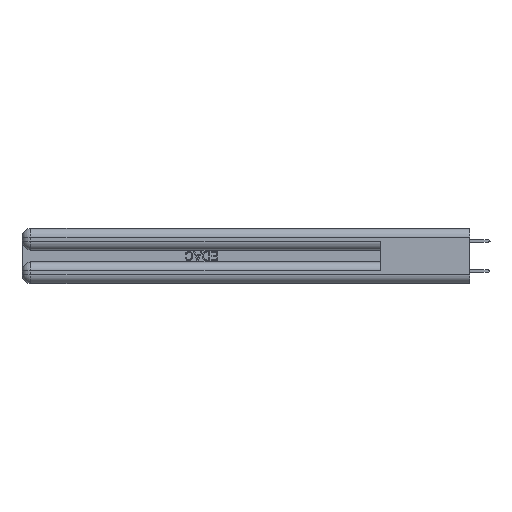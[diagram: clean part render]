
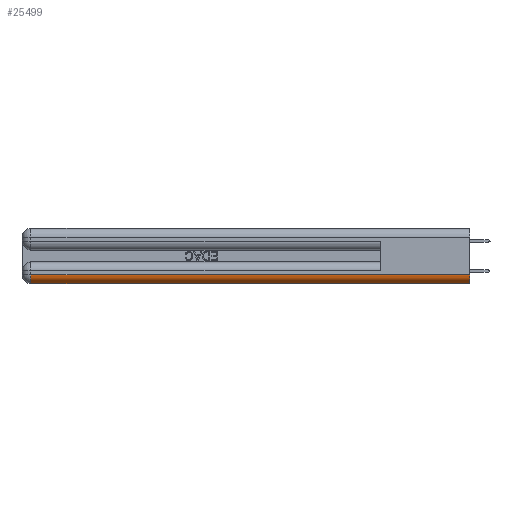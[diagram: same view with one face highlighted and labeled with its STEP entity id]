
A CAD part, left-side view. The second image highlights one B-rep face of the part: STEP entity #25499.
In plain terms, the highlighted cylindrical face has radius 1.524 mm (diameter 3.048 mm), a partial arc.
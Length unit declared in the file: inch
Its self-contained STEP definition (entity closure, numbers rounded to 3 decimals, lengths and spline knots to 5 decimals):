
#2619 = CIRCLE ( 'NONE', #36036, 0.06 ) ;
#3990 = EDGE_CURVE ( 'NONE', #31876, #46139, #46583, .T. ) ;
#4435 = FACE_OUTER_BOUND ( 'NONE', #39129, .T. ) ;
#6212 = EDGE_CURVE ( 'NONE', #35698, #48618, #12039, .T. ) ;
#7409 = DIRECTION ( 'NONE',  ( 0., 0., 1. ) ) ;
#9797 = CARTESIAN_POINT ( 'NONE',  ( 0.06, 2.94, 0. ) ) ;
#11845 = VECTOR ( 'NONE', #38698, 39.37008 ) ;
#12039 = LINE ( 'NONE', #42463, #11845 ) ;
#12673 = ORIENTED_EDGE ( 'NONE', *, *, #6212, .F. ) ;
#13856 = CARTESIAN_POINT ( 'NONE',  ( 0., 2.94, 0.06 ) ) ;
#14086 = VECTOR ( 'NONE', #35051, 39.37008 ) ;
#19617 = DIRECTION ( 'NONE',  ( 0., 1., 0. ) ) ;
#21204 = EDGE_CURVE ( 'NONE', #46139, #35698, #23054, .T. ) ;
#23054 = CIRCLE ( 'NONE', #31010, 0.06 ) ;
#23393 = ORIENTED_EDGE ( 'NONE', *, *, #3990, .F. ) ;
#25353 = DIRECTION ( 'NONE',  ( 0., 0., 1. ) ) ;
#25499 = ADVANCED_FACE ( 'NONE', ( #4435 ), #49086, .T. ) ;
#26378 = DIRECTION ( 'NONE',  ( 0., 0., 1. ) ) ;
#29340 = DIRECTION ( 'NONE',  ( 0., -1., 0. ) ) ;
#29714 = CARTESIAN_POINT ( 'NONE',  ( 0.06, 0., 0. ) ) ;
#30313 = EDGE_CURVE ( 'NONE', #48618, #31876, #2619, .T. ) ;
#30830 = CARTESIAN_POINT ( 'NONE',  ( 0., 0., 0.06 ) ) ;
#31010 = AXIS2_PLACEMENT_3D ( 'NONE', #41061, #29340, #25353 ) ;
#31876 = VERTEX_POINT ( 'NONE', #13856 ) ;
#32418 = ORIENTED_EDGE ( 'NONE', *, *, #30313, .F. ) ;
#32891 = AXIS2_PLACEMENT_3D ( 'NONE', #45591, #19617, #26378 ) ;
#35051 = DIRECTION ( 'NONE',  ( 0., -1., 0. ) ) ;
#35698 = VERTEX_POINT ( 'NONE', #29714 ) ;
#36036 = AXIS2_PLACEMENT_3D ( 'NONE', #45833, #37816, #7409 ) ;
#37117 = ORIENTED_EDGE ( 'NONE', *, *, #21204, .F. ) ;
#37816 = DIRECTION ( 'NONE',  ( 0., 1., 0. ) ) ;
#38698 = DIRECTION ( 'NONE',  ( 0., 1., 0. ) ) ;
#39129 = EDGE_LOOP ( 'NONE', ( #37117, #23393, #32418, #12673 ) ) ;
#41061 = CARTESIAN_POINT ( 'NONE',  ( 0.06, 0., 0.06 ) ) ;
#42463 = CARTESIAN_POINT ( 'NONE',  ( 0.06, 3., 0. ) ) ;
#45591 = CARTESIAN_POINT ( 'NONE',  ( 0.06, 0., 0.06 ) ) ;
#45833 = CARTESIAN_POINT ( 'NONE',  ( 0.06, 2.94, 0.06 ) ) ;
#46139 = VERTEX_POINT ( 'NONE', #48330 ) ;
#46583 = LINE ( 'NONE', #30830, #14086 ) ;
#48330 = CARTESIAN_POINT ( 'NONE',  ( 0., 0., 0.06 ) ) ;
#48618 = VERTEX_POINT ( 'NONE', #9797 ) ;
#49086 = CYLINDRICAL_SURFACE ( 'NONE', #32891, 0.06 ) ;
